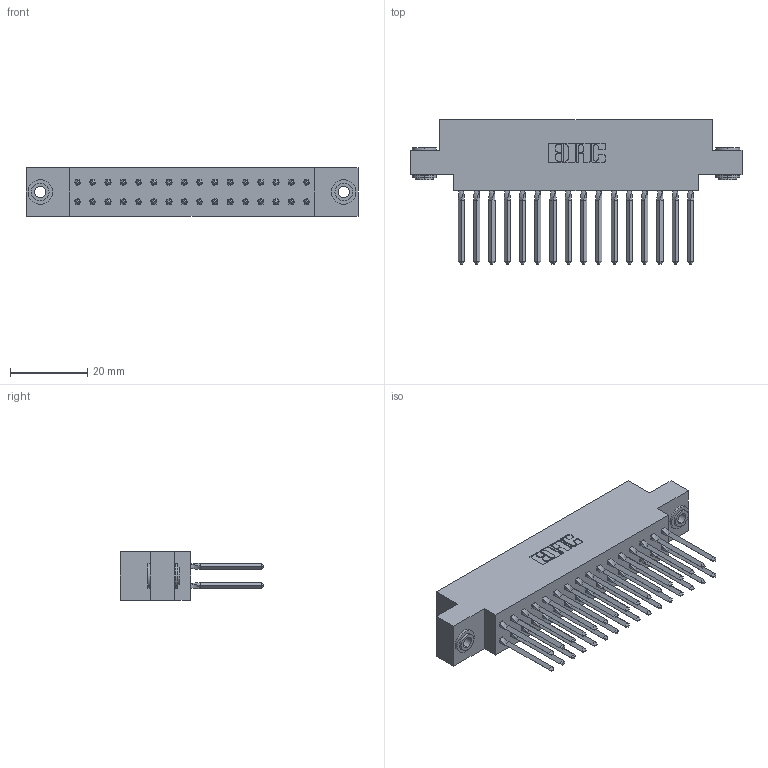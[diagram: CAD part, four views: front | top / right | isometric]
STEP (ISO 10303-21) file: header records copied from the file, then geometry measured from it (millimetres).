
FILE_DESCRIPTION (( 'STEP AP203' ), '1' );
FILE_NAME ('317-032-540-803.STEP', '2020-02-27T21:07:00', ( '' ), ( '' ), 'SwSTEP 2.0', 'SolidWorks 2016', '' );
FILE_SCHEMA (( 'CONFIG_CONTROL_DESIGN' ));
Length unit declared in the file: inch
Products named in the file (4): 317-032-540-803; 317-290-001_540; 317 Part_.156 Dia - TH; 345-250-002_345-250-002-102
Assembly tree (35 placements, depth 2):
  317-032-540-803
    317 Part_.156 Dia - TH
    317-290-001_540  x32
    345-250-002_345-250-002-102  x2
Bounding box: 86.11 x 37.34 x 12.7 mm (x, y, z)
Volume: 13591.6 mm3; surface area: 19495.1 mm2
Topology: 35 solids, 35 shells, 2988 faces, 8255 edges, 5318 vertices
Faces by surface type: plane 2404, cylinder 448, bspline 128, cone 8
Entity records: 27405 total; most frequent: CARTESIAN_POINT 5162, ORIENTED_EDGE 4654, DIRECTION 3927, EDGE_CURVE 2327, LINE 2047, VECTOR 2047, VERTEX_POINT 1543, AXIS2_PLACEMENT_3D 940
